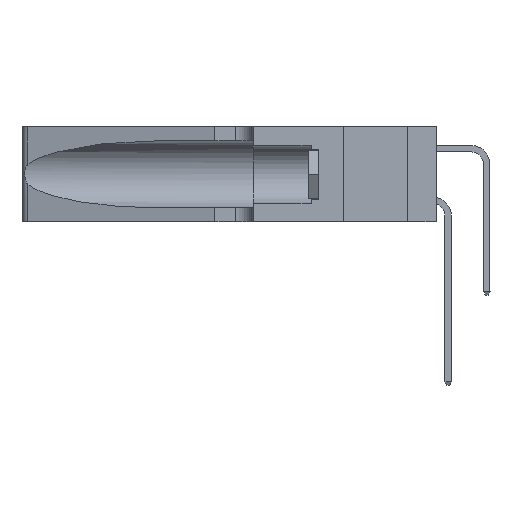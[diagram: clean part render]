
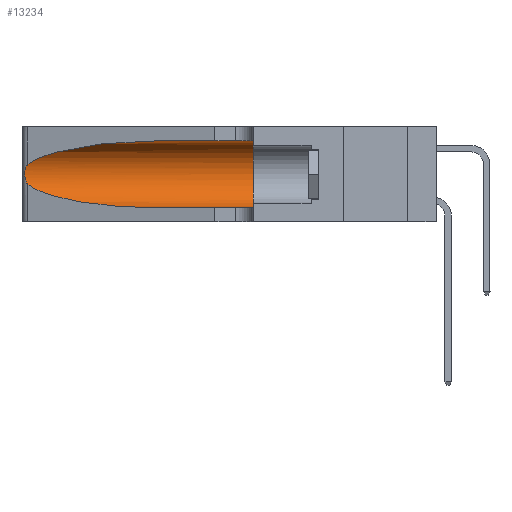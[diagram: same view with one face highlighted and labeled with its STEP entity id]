
A CAD part, left-side view. The second image highlights one B-rep face of the part: STEP entity #13234.
In plain terms, the highlighted cylindrical face has radius 3.308 mm (diameter 6.617 mm), a partial arc.
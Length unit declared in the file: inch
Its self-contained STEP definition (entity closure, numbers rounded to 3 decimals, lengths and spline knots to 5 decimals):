
#313 = VERTEX_POINT ( 'NONE', #22618 ) ;
#331 = ORIENTED_EDGE ( 'NONE', *, *, #28787, .T. ) ;
#677 = CARTESIAN_POINT ( 'NONE',  ( 0.25639, 1.23184, 0.21858 ) ) ;
#772 = DIRECTION ( 'NONE',  ( 0., 1., 0. ) ) ;
#802 = CARTESIAN_POINT ( 'NONE',  ( 0.25789, 1.23486, 0.15765 ) ) ;
#1694 = VECTOR ( 'NONE', #34436, 39.37008 ) ;
#2141 = CARTESIAN_POINT ( 'NONE',  ( 0.18966, 0.96281, 0.31525 ) ) ;
#2248 = LINE ( 'NONE', #17144, #7298 ) ;
#2904 = CARTESIAN_POINT ( 'NONE',  ( 0.18966, 0.96281, 0.05475 ) ) ;
#3349 = CARTESIAN_POINT ( 'NONE',  ( 0.25854, 1.2359, 0.20912 ) ) ;
#3797 = CARTESIAN_POINT ( 'NONE',  ( 0.25787, 1.23484, 0.2124 ) ) ;
#4294 = CARTESIAN_POINT ( 'NONE',  ( 0.1305, 1.61858, 0.185 ) ) ;
#5100 = CARTESIAN_POINT ( 'NONE',  ( 0.1305, 0.35, 0.31525 ) ) ;
#6057 = CYLINDRICAL_SURFACE ( 'NONE', #22251, 0.13025 ) ;
#6488 = CARTESIAN_POINT ( 'NONE',  ( 0.26075, 1.23896, 0.19203 ) ) ;
#7298 = VECTOR ( 'NONE', #22394, 39.37008 ) ;
#7568 = ORIENTED_EDGE ( 'NONE', *, *, #24609, .T. ) ;
#7570 = CARTESIAN_POINT ( 'NONE',  ( 0.2373, 1.15595, 0.28018 ) ) ;
#7794 = CARTESIAN_POINT ( 'NONE',  ( 0.1305, 0.72297, 0.31525 ) ) ;
#8035 = B_SPLINE_CURVE_WITH_KNOTS ( 'NONE', 3,
 ( #16979, #30331, #677, #3797, #3349, #8609, #6488, #14028, #8831, #27519, #802, #14247, #11315, #27623 ),
 .UNSPECIFIED., .F., .F.,
 ( 4, 2, 2, 2, 2, 2, 4 ),
 ( 0., 0.00027, 0.00053, 0.00107, 0.0016, 0.00187, 0.00214 ),
 .UNSPECIFIED. ) ;
#8609 = CARTESIAN_POINT ( 'NONE',  ( 0.26018, 1.23835, 0.19895 ) ) ;
#8810 = CARTESIAN_POINT ( 'NONE',  ( 0.1305, 0.72297, 0.05475 ) ) ;
#8812 = CARTESIAN_POINT ( 'NONE',  ( 0.1305, 0.35, 0.185 ) ) ;
#8831 = CARTESIAN_POINT ( 'NONE',  ( 0.26017, 1.23833, 0.17102 ) ) ;
#11315 = CARTESIAN_POINT ( 'NONE',  ( 0.25555, 1.22993, 0.14849 ) ) ;
#11667 = VERTEX_POINT ( 'NONE', #5100 ) ;
#12411 = FACE_OUTER_BOUND ( 'NONE', #23200, .T. ) ;
#13117 = LINE ( 'NONE', #31320, #1694 ) ;
#13234 = ADVANCED_FACE ( 'NONE', ( #12411 ), #6057, .F. ) ;
#14028 = CARTESIAN_POINT ( 'NONE',  ( 0.26075, 1.23896, 0.178 ) ) ;
#14171 = EDGE_CURVE ( 'NONE', #29615, #18952, #2248, .T. ) ;
#14247 = CARTESIAN_POINT ( 'NONE',  ( 0.25639, 1.23186, 0.15144 ) ) ;
#15696 = CARTESIAN_POINT ( 'NONE',  ( 0.25487, 1.22718, 0.22369 ) ) ;
#16421 =( BOUNDED_CURVE ( )  B_SPLINE_CURVE ( 3, ( #7794, #2141, #7570, #15696 ),
 .UNSPECIFIED., .F., .F. ) 
 B_SPLINE_CURVE_WITH_KNOTS ( ( 4, 4 ),
 ( 1.5708, 2.84003 ),
 .UNSPECIFIED. ) 
 CURVE ( )  GEOMETRIC_REPRESENTATION_ITEM ( )  RATIONAL_B_SPLINE_CURVE ( ( 1., 0.87, 0.87, 1. ) ) 
 REPRESENTATION_ITEM ( '' )  );
#16839 = CARTESIAN_POINT ( 'NONE',  ( 0.25487, 1.22718, 0.14631 ) ) ;
#16979 = CARTESIAN_POINT ( 'NONE',  ( 0.25487, 1.22718, 0.22369 ) ) ;
#17144 = CARTESIAN_POINT ( 'NONE',  ( 0.1305, 1.61858, 0.05475 ) ) ;
#18952 = VERTEX_POINT ( 'NONE', #22666 ) ;
#19211 = AXIS2_PLACEMENT_3D ( 'NONE', #8812, #772, #33052 ) ;
#20340 = CIRCLE ( 'NONE', #19211, 0.13025 ) ;
#20736 = CARTESIAN_POINT ( 'NONE',  ( 0.1305, 0.72297, 0.05475 ) ) ;
#20814 = ORIENTED_EDGE ( 'NONE', *, *, #30485, .F. ) ;
#22251 = AXIS2_PLACEMENT_3D ( 'NONE', #4294, #26350, #23199 ) ;
#22274 = EDGE_CURVE ( 'NONE', #11667, #18952, #20340, .T. ) ;
#22360 = EDGE_CURVE ( 'NONE', #26671, #29615, #34248, .T. ) ;
#22394 = DIRECTION ( 'NONE',  ( 0., -1., 0. ) ) ;
#22618 = CARTESIAN_POINT ( 'NONE',  ( 0.1305, 0.72297, 0.31525 ) ) ;
#22647 = CARTESIAN_POINT ( 'NONE',  ( 0.25487, 1.22718, 0.14631 ) ) ;
#22666 = CARTESIAN_POINT ( 'NONE',  ( 0.1305, 0.35, 0.05475 ) ) ;
#23199 = DIRECTION ( 'NONE',  ( 0., 0., -1. ) ) ;
#23200 = EDGE_LOOP ( 'NONE', ( #7568, #331, #31061, #29637, #26660, #20814 ) ) ;
#23873 = VERTEX_POINT ( 'NONE', #24135 ) ;
#24135 = CARTESIAN_POINT ( 'NONE',  ( 0.25487, 1.22718, 0.22369 ) ) ;
#24609 = EDGE_CURVE ( 'NONE', #313, #23873, #16421, .T. ) ;
#26350 = DIRECTION ( 'NONE',  ( 0., -1., 0. ) ) ;
#26660 = ORIENTED_EDGE ( 'NONE', *, *, #22274, .F. ) ;
#26671 = VERTEX_POINT ( 'NONE', #22647 ) ;
#27519 = CARTESIAN_POINT ( 'NONE',  ( 0.25856, 1.23593, 0.16098 ) ) ;
#27623 = CARTESIAN_POINT ( 'NONE',  ( 0.25487, 1.22718, 0.14631 ) ) ;
#28787 = EDGE_CURVE ( 'NONE', #23873, #26671, #8035, .T. ) ;
#29615 = VERTEX_POINT ( 'NONE', #20736 ) ;
#29637 = ORIENTED_EDGE ( 'NONE', *, *, #14171, .T. ) ;
#29798 = CARTESIAN_POINT ( 'NONE',  ( 0.2373, 1.15595, 0.08982 ) ) ;
#30331 = CARTESIAN_POINT ( 'NONE',  ( 0.25555, 1.22994, 0.2215 ) ) ;
#30485 = EDGE_CURVE ( 'NONE', #313, #11667, #13117, .T. ) ;
#31061 = ORIENTED_EDGE ( 'NONE', *, *, #22360, .T. ) ;
#31320 = CARTESIAN_POINT ( 'NONE',  ( 0.1305, 1.61858, 0.31525 ) ) ;
#33052 = DIRECTION ( 'NONE',  ( 0., 0., 1. ) ) ;
#34248 =( BOUNDED_CURVE ( )  B_SPLINE_CURVE ( 3, ( #16839, #29798, #2904, #8810 ),
 .UNSPECIFIED., .F., .F. ) 
 B_SPLINE_CURVE_WITH_KNOTS ( ( 4, 4 ),
 ( 3.44316, 4.71239 ),
 .UNSPECIFIED. ) 
 CURVE ( )  GEOMETRIC_REPRESENTATION_ITEM ( )  RATIONAL_B_SPLINE_CURVE ( ( 1., 0.87, 0.87, 1. ) ) 
 REPRESENTATION_ITEM ( '' )  );
#34436 = DIRECTION ( 'NONE',  ( 0., -1., 0. ) ) ;
